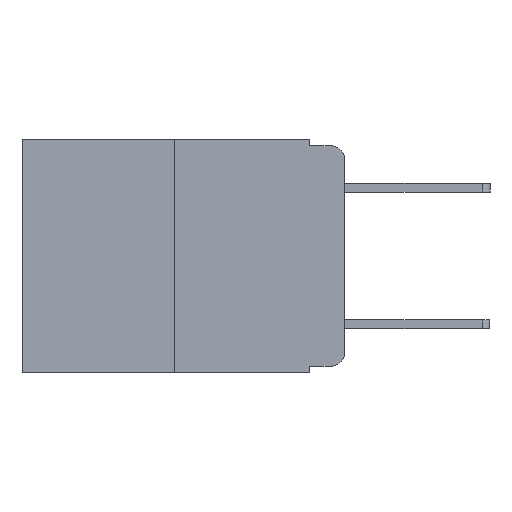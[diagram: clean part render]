
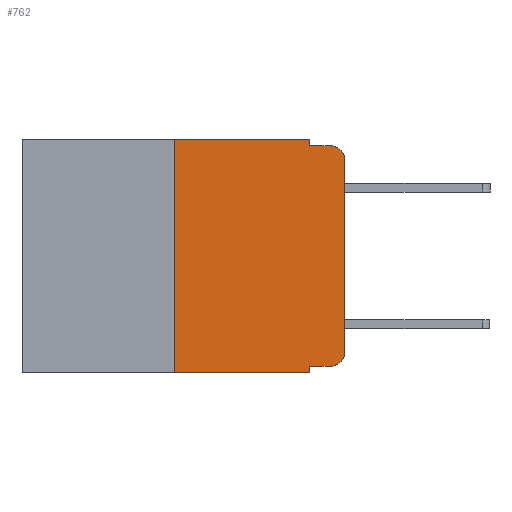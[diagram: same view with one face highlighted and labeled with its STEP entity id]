
A CAD part, left-side view. The second image highlights one B-rep face of the part: STEP entity #762.
In plain terms, the highlighted planar face has unit normal (-1, 0, 0).
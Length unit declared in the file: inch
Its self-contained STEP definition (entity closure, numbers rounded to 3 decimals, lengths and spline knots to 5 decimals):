
#241 = VECTOR ( 'NONE', #7763, 39.37008 ) ;
#378 = CARTESIAN_POINT ( 'NONE',  ( 0., 0.473, -0.343 ) ) ;
#473 = VECTOR ( 'NONE', #14039, 39.37008 ) ;
#762 = ADVANCED_FACE ( 'NONE', ( #21152 ), #13645, .F. ) ;
#1110 = DIRECTION ( 'NONE',  ( 0., 0., -1. ) ) ;
#1414 = VERTEX_POINT ( 'NONE', #13489 ) ;
#1501 = ORIENTED_EDGE ( 'NONE', *, *, #17719, .T. ) ;
#1569 = ORIENTED_EDGE ( 'NONE', *, *, #14587, .F. ) ;
#1639 = ORIENTED_EDGE ( 'NONE', *, *, #15875, .T. ) ;
#2174 = VECTOR ( 'NONE', #17853, 39.37008 ) ;
#2451 = VERTEX_POINT ( 'NONE', #15130 ) ;
#2567 = VERTEX_POINT ( 'NONE', #3666 ) ;
#2758 = LINE ( 'NONE', #16269, #2174 ) ;
#3053 = ORIENTED_EDGE ( 'NONE', *, *, #7138, .T. ) ;
#3144 = CARTESIAN_POINT ( 'NONE',  ( 0., 0.051, -0.01 ) ) ;
#3217 = VECTOR ( 'NONE', #5084, 39.37008 ) ;
#3307 = CARTESIAN_POINT ( 'NONE',  ( 0., 0.051, 0. ) ) ;
#3453 = VECTOR ( 'NONE', #20030, 39.37008 ) ;
#3666 = CARTESIAN_POINT ( 'NONE',  ( 0., 0.051, -0.343 ) ) ;
#3753 = VECTOR ( 'NONE', #13337, 39.37008 ) ;
#4286 = CARTESIAN_POINT ( 'NONE',  ( 0., 0.473, 0. ) ) ;
#4533 = VERTEX_POINT ( 'NONE', #20081 ) ;
#4639 = EDGE_LOOP ( 'NONE', ( #6026, #1501, #11978, #1569, #5250, #16694, #1639, #15007, #14534, #3053 ) ) ;
#5084 = DIRECTION ( 'NONE',  ( 0., 0., -1. ) ) ;
#5250 = ORIENTED_EDGE ( 'NONE', *, *, #8054, .F. ) ;
#6026 = ORIENTED_EDGE ( 'NONE', *, *, #19751, .T. ) ;
#6124 = CARTESIAN_POINT ( 'NONE',  ( 0., 0.473, 0. ) ) ;
#6369 = DIRECTION ( 'NONE',  ( 0., 0., -1. ) ) ;
#6382 = CARTESIAN_POINT ( 'NONE',  ( 0., 0., -0.03 ) ) ;
#7024 = CARTESIAN_POINT ( 'NONE',  ( 0., 0.051, -0.01 ) ) ;
#7033 = AXIS2_PLACEMENT_3D ( 'NONE', #7982, #18952, #9683 ) ;
#7138 = EDGE_CURVE ( 'NONE', #17046, #2451, #20046, .T. ) ;
#7763 = DIRECTION ( 'NONE',  ( 0., -1., 0. ) ) ;
#7982 = CARTESIAN_POINT ( 'NONE',  ( 0., 0.02, -0.03 ) ) ;
#8054 = EDGE_CURVE ( 'NONE', #1414, #20529, #9655, .T. ) ;
#8253 = EDGE_CURVE ( 'NONE', #16463, #17046, #9402, .T. ) ;
#8384 = CARTESIAN_POINT ( 'NONE',  ( 0., 0.02, -0.333 ) ) ;
#8854 = CARTESIAN_POINT ( 'NONE',  ( 0., 0.25, -0.343 ) ) ;
#9402 = LINE ( 'NONE', #10136, #13481 ) ;
#9655 = LINE ( 'NONE', #6124, #241 ) ;
#9683 = DIRECTION ( 'NONE',  ( 0., 0., -1. ) ) ;
#10136 = CARTESIAN_POINT ( 'NONE',  ( 0., 0.051, -0.333 ) ) ;
#10452 = DIRECTION ( 'NONE',  ( 1., 0., 0. ) ) ;
#11324 = DIRECTION ( 'NONE',  ( -1., 0., 0. ) ) ;
#11978 = ORIENTED_EDGE ( 'NONE', *, *, #15617, .F. ) ;
#12023 = VECTOR ( 'NONE', #19046, 39.37008 ) ;
#12482 = EDGE_CURVE ( 'NONE', #16463, #2567, #2758, .T. ) ;
#12511 = LINE ( 'NONE', #17503, #12023 ) ;
#12672 = VERTEX_POINT ( 'NONE', #8854 ) ;
#13337 = DIRECTION ( 'NONE',  ( 0., -1., 0. ) ) ;
#13481 = VECTOR ( 'NONE', #19395, 39.37008 ) ;
#13489 = CARTESIAN_POINT ( 'NONE',  ( 0., 0.25, 0. ) ) ;
#13501 = EDGE_CURVE ( 'NONE', #12672, #1414, #12511, .T. ) ;
#13645 = PLANE ( 'NONE',  #15353 ) ;
#14039 = DIRECTION ( 'NONE',  ( 0., 0., 1. ) ) ;
#14534 = ORIENTED_EDGE ( 'NONE', *, *, #8253, .T. ) ;
#14587 = EDGE_CURVE ( 'NONE', #20529, #19277, #16128, .T. ) ;
#14973 = CIRCLE ( 'NONE', #7033, 0.02 ) ;
#15007 = ORIENTED_EDGE ( 'NONE', *, *, #12482, .F. ) ;
#15130 = CARTESIAN_POINT ( 'NONE',  ( 0., 0., -0.313 ) ) ;
#15353 = AXIS2_PLACEMENT_3D ( 'NONE', #4286, #10452, #6369 ) ;
#15617 = EDGE_CURVE ( 'NONE', #19277, #4533, #20660, .T. ) ;
#15875 = EDGE_CURVE ( 'NONE', #12672, #2567, #20411, .T. ) ;
#16128 = LINE ( 'NONE', #3307, #3217 ) ;
#16163 = AXIS2_PLACEMENT_3D ( 'NONE', #20568, #11324, #1110 ) ;
#16269 = CARTESIAN_POINT ( 'NONE',  ( 0., 0.051, 0. ) ) ;
#16463 = VERTEX_POINT ( 'NONE', #20928 ) ;
#16694 = ORIENTED_EDGE ( 'NONE', *, *, #13501, .F. ) ;
#17046 = VERTEX_POINT ( 'NONE', #8384 ) ;
#17503 = CARTESIAN_POINT ( 'NONE',  ( 0., 0.25, 0. ) ) ;
#17719 = EDGE_CURVE ( 'NONE', #19914, #4533, #14973, .T. ) ;
#17853 = DIRECTION ( 'NONE',  ( 0., 0., -1. ) ) ;
#18064 = LINE ( 'NONE', #20174, #473 ) ;
#18903 = CARTESIAN_POINT ( 'NONE',  ( 0., 0.051, 0. ) ) ;
#18952 = DIRECTION ( 'NONE',  ( -1., 0., 0. ) ) ;
#19046 = DIRECTION ( 'NONE',  ( 0., 0., 1. ) ) ;
#19277 = VERTEX_POINT ( 'NONE', #3144 ) ;
#19395 = DIRECTION ( 'NONE',  ( 0., -1., 0. ) ) ;
#19751 = EDGE_CURVE ( 'NONE', #2451, #19914, #18064, .T. ) ;
#19914 = VERTEX_POINT ( 'NONE', #6382 ) ;
#20030 = DIRECTION ( 'NONE',  ( 0., -1., 0. ) ) ;
#20046 = CIRCLE ( 'NONE', #16163, 0.02 ) ;
#20081 = CARTESIAN_POINT ( 'NONE',  ( 0., 0.02, -0.01 ) ) ;
#20174 = CARTESIAN_POINT ( 'NONE',  ( 0., 0., 0. ) ) ;
#20411 = LINE ( 'NONE', #378, #3453 ) ;
#20529 = VERTEX_POINT ( 'NONE', #18903 ) ;
#20568 = CARTESIAN_POINT ( 'NONE',  ( 0., 0.02, -0.313 ) ) ;
#20660 = LINE ( 'NONE', #7024, #3753 ) ;
#20928 = CARTESIAN_POINT ( 'NONE',  ( 0., 0.051, -0.333 ) ) ;
#21152 = FACE_OUTER_BOUND ( 'NONE', #4639, .T. ) ;
